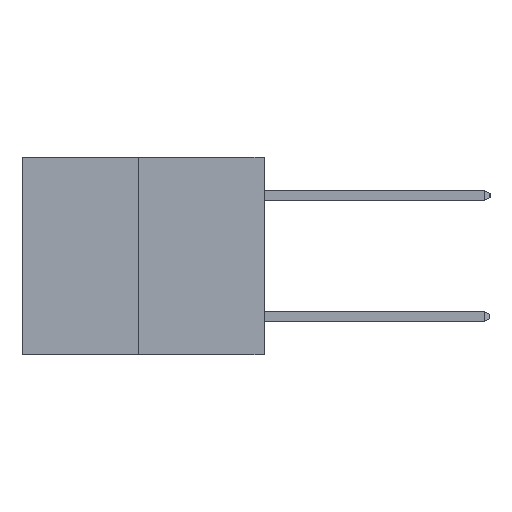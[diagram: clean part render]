
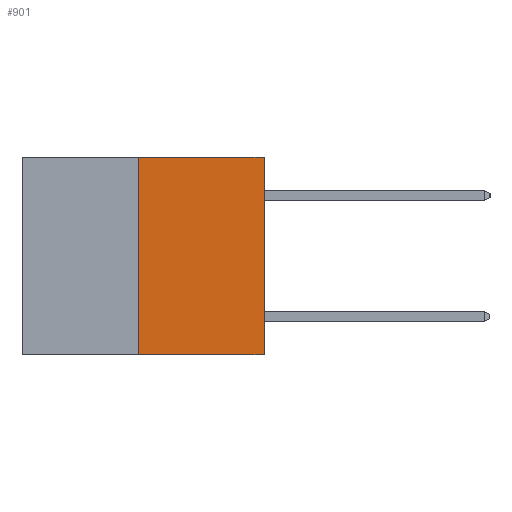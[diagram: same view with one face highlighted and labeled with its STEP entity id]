
A CAD part, left-side view. The second image highlights one B-rep face of the part: STEP entity #901.
In plain terms, the highlighted planar face has unit normal (-1, 0, 0).
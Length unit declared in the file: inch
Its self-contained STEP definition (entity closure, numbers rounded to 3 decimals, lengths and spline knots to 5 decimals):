
#646 = EDGE_LOOP ( 'NONE', ( #4302, #1474, #10851, #5652 ) ) ;
#901 = ADVANCED_FACE ( 'NONE', ( #1251 ), #11818, .F. ) ;
#996 = DIRECTION ( 'NONE',  ( 0., 0., 1. ) ) ;
#1251 = FACE_OUTER_BOUND ( 'NONE', #646, .T. ) ;
#1385 = VECTOR ( 'NONE', #6613, 39.37008 ) ;
#1474 = ORIENTED_EDGE ( 'NONE', *, *, #1627, .T. ) ;
#1539 = VECTOR ( 'NONE', #9648, 39.37008 ) ;
#1627 = EDGE_CURVE ( 'NONE', #5221, #1923, #8533, .T. ) ;
#1923 = VERTEX_POINT ( 'NONE', #4556 ) ;
#2104 = AXIS2_PLACEMENT_3D ( 'NONE', #6155, #3976, #11493 ) ;
#3145 = VECTOR ( 'NONE', #996, 39.37008 ) ;
#3357 = LINE ( 'NONE', #3783, #11529 ) ;
#3578 = LINE ( 'NONE', #6566, #3145 ) ;
#3650 = CARTESIAN_POINT ( 'NONE',  ( 0., 0.312, 0. ) ) ;
#3783 = CARTESIAN_POINT ( 'NONE',  ( 0., 0.6, 0. ) ) ;
#3976 = DIRECTION ( 'NONE',  ( 1., 0., 0. ) ) ;
#4302 = ORIENTED_EDGE ( 'NONE', *, *, #12278, .F. ) ;
#4556 = CARTESIAN_POINT ( 'NONE',  ( 0., 0., -0.49 ) ) ;
#5221 = VERTEX_POINT ( 'NONE', #10586 ) ;
#5529 = EDGE_CURVE ( 'NONE', #1923, #11306, #3578, .T. ) ;
#5597 = CARTESIAN_POINT ( 'NONE',  ( 0., 0.6, -0.49 ) ) ;
#5652 = ORIENTED_EDGE ( 'NONE', *, *, #11856, .F. ) ;
#6155 = CARTESIAN_POINT ( 'NONE',  ( 0., 0.6, 0. ) ) ;
#6566 = CARTESIAN_POINT ( 'NONE',  ( 0., 0., 0. ) ) ;
#6613 = DIRECTION ( 'NONE',  ( 0., -1., 0. ) ) ;
#7822 = CARTESIAN_POINT ( 'NONE',  ( 0., 0.312, -0.49 ) ) ;
#8533 = LINE ( 'NONE', #5597, #1385 ) ;
#9286 = LINE ( 'NONE', #7822, #1539 ) ;
#9648 = DIRECTION ( 'NONE',  ( 0., 0., 1. ) ) ;
#10586 = CARTESIAN_POINT ( 'NONE',  ( 0., 0.312, -0.49 ) ) ;
#10618 = DIRECTION ( 'NONE',  ( 0., -1., 0. ) ) ;
#10851 = ORIENTED_EDGE ( 'NONE', *, *, #5529, .T. ) ;
#11072 = VERTEX_POINT ( 'NONE', #3650 ) ;
#11306 = VERTEX_POINT ( 'NONE', #11534 ) ;
#11493 = DIRECTION ( 'NONE',  ( 0., 0., -1. ) ) ;
#11529 = VECTOR ( 'NONE', #10618, 39.37008 ) ;
#11534 = CARTESIAN_POINT ( 'NONE',  ( 0., 0., 0. ) ) ;
#11818 = PLANE ( 'NONE',  #2104 ) ;
#11856 = EDGE_CURVE ( 'NONE', #11072, #11306, #3357, .T. ) ;
#12278 = EDGE_CURVE ( 'NONE', #5221, #11072, #9286, .T. ) ;
